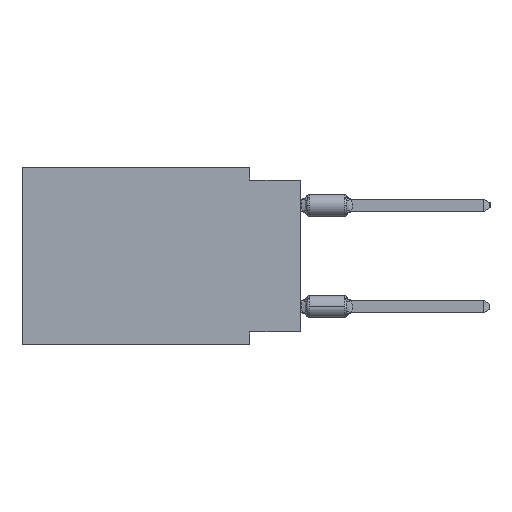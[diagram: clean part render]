
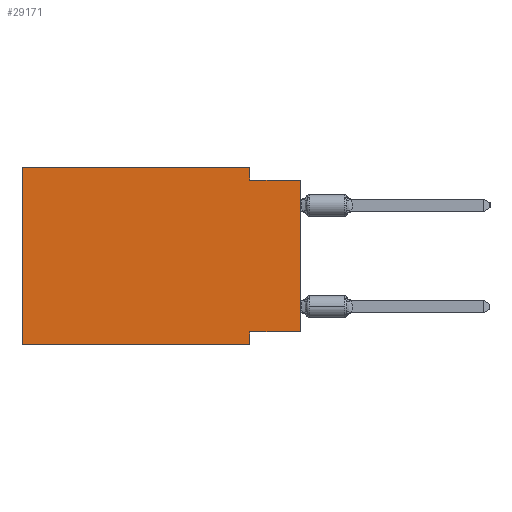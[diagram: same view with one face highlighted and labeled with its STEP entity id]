
A CAD part, left-side view. The second image highlights one B-rep face of the part: STEP entity #29171.
In plain terms, the highlighted planar face has unit normal (-1, 0, 0).
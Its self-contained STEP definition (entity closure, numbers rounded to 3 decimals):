
#987 = CARTESIAN_POINT ( 'NONE',  ( 0., 2.54, -8.255 ) ) ;
#1313 = VECTOR ( 'NONE', #23234, 1000. ) ;
#2126 = ORIENTED_EDGE ( 'NONE', *, *, #20011, .T. ) ;
#2140 = VERTEX_POINT ( 'NONE', #987 ) ;
#2350 = CARTESIAN_POINT ( 'NONE',  ( 0., 2.54, -0.635 ) ) ;
#3637 = DIRECTION ( 'NONE',  ( 0., -1., 0. ) ) ;
#4051 = LINE ( 'NONE', #26778, #6543 ) ;
#4215 = CARTESIAN_POINT ( 'NONE',  ( 0., 2.54, 0. ) ) ;
#5336 = VERTEX_POINT ( 'NONE', #2350 ) ;
#5460 = CARTESIAN_POINT ( 'NONE',  ( 0., 0., -0.635 ) ) ;
#5761 = VECTOR ( 'NONE', #21823, 1000. ) ;
#5780 = CARTESIAN_POINT ( 'NONE',  ( 0., 2.54, 0. ) ) ;
#6543 = VECTOR ( 'NONE', #31552, 1000. ) ;
#6777 = CARTESIAN_POINT ( 'NONE',  ( 0., 13.97, 0. ) ) ;
#7352 = CARTESIAN_POINT ( 'NONE',  ( 0., 0., -8.255 ) ) ;
#8940 = ORIENTED_EDGE ( 'NONE', *, *, #20585, .F. ) ;
#9234 = CARTESIAN_POINT ( 'NONE',  ( 0., 0., 0. ) ) ;
#9564 = LINE ( 'NONE', #6777, #9950 ) ;
#9653 = EDGE_CURVE ( 'NONE', #12312, #31322, #9564, .T. ) ;
#9950 = VECTOR ( 'NONE', #17139, 1000. ) ;
#10287 = FACE_OUTER_BOUND ( 'NONE', #30785, .T. ) ;
#11455 = VERTEX_POINT ( 'NONE', #17343 ) ;
#11531 = VECTOR ( 'NONE', #17640, 1000. ) ;
#11705 = ORIENTED_EDGE ( 'NONE', *, *, #21477, .F. ) ;
#12075 = EDGE_CURVE ( 'NONE', #12189, #2140, #4051, .T. ) ;
#12087 = VECTOR ( 'NONE', #24378, 1000. ) ;
#12189 = VERTEX_POINT ( 'NONE', #7352 ) ;
#12312 = VERTEX_POINT ( 'NONE', #17860 ) ;
#12588 = ORIENTED_EDGE ( 'NONE', *, *, #12750, .F. ) ;
#12750 = EDGE_CURVE ( 'NONE', #5336, #25611, #12876, .T. ) ;
#12876 = LINE ( 'NONE', #5460, #1313 ) ;
#12944 = DIRECTION ( 'NONE',  ( 0., 0., -1. ) ) ;
#13412 = CARTESIAN_POINT ( 'NONE',  ( 0., 13.97, 0. ) ) ;
#14859 = LINE ( 'NONE', #27211, #11531 ) ;
#15237 = AXIS2_PLACEMENT_3D ( 'NONE', #13412, #18025, #18346 ) ;
#16009 = ORIENTED_EDGE ( 'NONE', *, *, #9653, .F. ) ;
#16814 = LINE ( 'NONE', #26522, #21561 ) ;
#16817 = LINE ( 'NONE', #9234, #12087 ) ;
#17139 = DIRECTION ( 'NONE',  ( 0., 0., 1. ) ) ;
#17343 = CARTESIAN_POINT ( 'NONE',  ( 0., 2.54, -8.89 ) ) ;
#17640 = DIRECTION ( 'NONE',  ( 0., -1., 0. ) ) ;
#17860 = CARTESIAN_POINT ( 'NONE',  ( 0., 13.97, -8.89 ) ) ;
#18025 = DIRECTION ( 'NONE',  ( 1., 0., 0. ) ) ;
#18066 = CARTESIAN_POINT ( 'NONE',  ( 0., 13.97, 0. ) ) ;
#18346 = DIRECTION ( 'NONE',  ( 0., 0., -1. ) ) ;
#18407 = ORIENTED_EDGE ( 'NONE', *, *, #12075, .F. ) ;
#19179 = EDGE_CURVE ( 'NONE', #2140, #11455, #29751, .T. ) ;
#20011 = EDGE_CURVE ( 'NONE', #12312, #11455, #14859, .T. ) ;
#20490 = PLANE ( 'NONE',  #15237 ) ;
#20585 = EDGE_CURVE ( 'NONE', #23051, #5336, #27096, .T. ) ;
#20909 = ORIENTED_EDGE ( 'NONE', *, *, #28609, .T. ) ;
#21477 = EDGE_CURVE ( 'NONE', #31322, #23051, #16814, .T. ) ;
#21561 = VECTOR ( 'NONE', #3637, 1000. ) ;
#21823 = DIRECTION ( 'NONE',  ( 0., 0., -1. ) ) ;
#23051 = VERTEX_POINT ( 'NONE', #5780 ) ;
#23234 = DIRECTION ( 'NONE',  ( 0., -1., 0. ) ) ;
#23551 = CARTESIAN_POINT ( 'NONE',  ( 0., 0., -0.635 ) ) ;
#24378 = DIRECTION ( 'NONE',  ( 0., 0., 1. ) ) ;
#25611 = VERTEX_POINT ( 'NONE', #23551 ) ;
#26522 = CARTESIAN_POINT ( 'NONE',  ( 0., 13.97, 0. ) ) ;
#26778 = CARTESIAN_POINT ( 'NONE',  ( 0., 0., -8.255 ) ) ;
#27096 = LINE ( 'NONE', #4215, #5761 ) ;
#27211 = CARTESIAN_POINT ( 'NONE',  ( 0., 13.97, -8.89 ) ) ;
#28609 = EDGE_CURVE ( 'NONE', #12189, #25611, #16817, .T. ) ;
#29171 = ADVANCED_FACE ( 'NONE', ( #10287 ), #20490, .F. ) ;
#29376 = ORIENTED_EDGE ( 'NONE', *, *, #19179, .F. ) ;
#29751 = LINE ( 'NONE', #30073, #31968 ) ;
#30073 = CARTESIAN_POINT ( 'NONE',  ( 0., 2.54, -8.89 ) ) ;
#30785 = EDGE_LOOP ( 'NONE', ( #20909, #12588, #8940, #11705, #16009, #2126, #29376, #18407 ) ) ;
#31322 = VERTEX_POINT ( 'NONE', #18066 ) ;
#31552 = DIRECTION ( 'NONE',  ( 0., 1., 0. ) ) ;
#31968 = VECTOR ( 'NONE', #12944, 1000. ) ;
